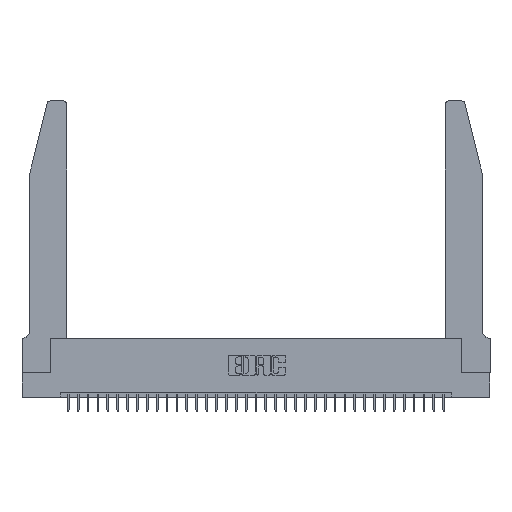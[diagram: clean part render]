
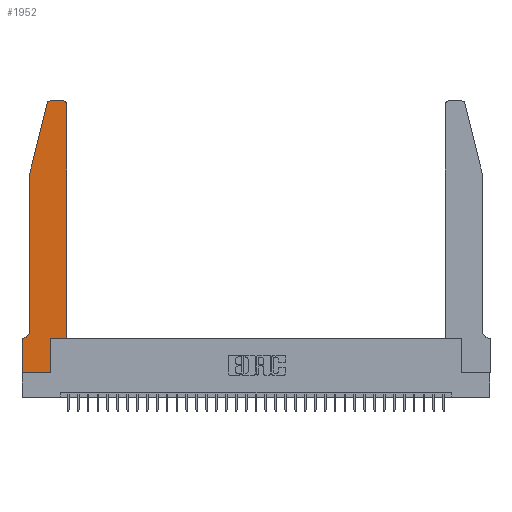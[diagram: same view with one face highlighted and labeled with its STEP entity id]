
A CAD part, top view. The second image highlights one B-rep face of the part: STEP entity #1952.
In plain terms, the highlighted planar face has unit normal (0, 0, 1).
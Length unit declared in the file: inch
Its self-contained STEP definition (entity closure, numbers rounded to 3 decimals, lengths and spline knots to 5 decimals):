
#158 = DIRECTION ( 'NONE',  ( 0., 0., -1. ) ) ;
#1492 = VECTOR ( 'NONE', #25824, 39.37008 ) ;
#1546 = CARTESIAN_POINT ( 'NONE',  ( 0.4505, 0.35, 0.37 ) ) ;
#1723 = LINE ( 'NONE', #1546, #2317 ) ;
#1856 = AXIS2_PLACEMENT_3D ( 'NONE', #34117, #3995, #17413 ) ;
#1952 = ADVANCED_FACE ( 'NONE', ( #29750 ), #30440, .T. ) ;
#2241 = DIRECTION ( 'NONE',  ( -1., 0., 0. ) ) ;
#2317 = VECTOR ( 'NONE', #34607, 39.37008 ) ;
#2616 = EDGE_CURVE ( 'NONE', #30620, #25859, #33422, .T. ) ;
#2762 = AXIS2_PLACEMENT_3D ( 'NONE', #13038, #24094, #8824 ) ;
#3745 = EDGE_CURVE ( 'NONE', #15324, #7167, #34876, .T. ) ;
#3892 = ORIENTED_EDGE ( 'NONE', *, *, #27287, .T. ) ;
#3995 = DIRECTION ( 'NONE',  ( 0., 0., 1. ) ) ;
#4018 = ORIENTED_EDGE ( 'NONE', *, *, #30330, .T. ) ;
#4283 = DIRECTION ( 'NONE',  ( 0., -1., 0. ) ) ;
#4850 = VERTEX_POINT ( 'NONE', #19926 ) ;
#4927 = CARTESIAN_POINT ( 'NONE',  ( 0.0055, 0.35, 0.37 ) ) ;
#5542 = DIRECTION ( 'NONE',  ( 0., 0., 1. ) ) ;
#5621 = DIRECTION ( 'NONE',  ( 0., 1., 0. ) ) ;
#5966 = DIRECTION ( 'NONE',  ( -1., 0., 0. ) ) ;
#6791 = CARTESIAN_POINT ( 'NONE',  ( 0.4505, 0.35, 0.37 ) ) ;
#7167 = VERTEX_POINT ( 'NONE', #4927 ) ;
#7569 = VECTOR ( 'NONE', #5621, 39.37008 ) ;
#8710 = CARTESIAN_POINT ( 'NONE',  ( 0.0755, 2., 0.37 ) ) ;
#8824 = DIRECTION ( 'NONE',  ( 1., 0., 0. ) ) ;
#9151 = CARTESIAN_POINT ( 'NONE',  ( 0., 0.35, 0.37 ) ) ;
#9332 = DIRECTION ( 'NONE',  ( 1., 0., 0. ) ) ;
#10185 = VECTOR ( 'NONE', #24872, 39.37008 ) ;
#10247 = ORIENTED_EDGE ( 'NONE', *, *, #20597, .T. ) ;
#10715 = EDGE_CURVE ( 'NONE', #7167, #22431, #14595, .T. ) ;
#11052 = VECTOR ( 'NONE', #28286, 39.37008 ) ;
#11178 = CARTESIAN_POINT ( 'NONE',  ( 0.25487, 2.72718, 0.37 ) ) ;
#11275 = CARTESIAN_POINT ( 'NONE',  ( 0.0755, 0.42, 0.37 ) ) ;
#13038 = CARTESIAN_POINT ( 'NONE',  ( 0.4205, 2.72, 0.37 ) ) ;
#14363 = CARTESIAN_POINT ( 'NONE',  ( 0.2865, 0.35, 0.37 ) ) ;
#14595 = LINE ( 'NONE', #31275, #1492 ) ;
#14712 = CARTESIAN_POINT ( 'NONE',  ( 0.284, 2.75, 0.37 ) ) ;
#14796 = CARTESIAN_POINT ( 'NONE',  ( 0., 0., 0.37 ) ) ;
#15324 = VERTEX_POINT ( 'NONE', #11275 ) ;
#15760 = VECTOR ( 'NONE', #2241, 39.37008 ) ;
#16419 = LINE ( 'NONE', #29851, #15760 ) ;
#16711 = EDGE_CURVE ( 'NONE', #26200, #34934, #25605, .T. ) ;
#16715 = ORIENTED_EDGE ( 'NONE', *, *, #2616, .T. ) ;
#16938 = CARTESIAN_POINT ( 'NONE',  ( 0.2865, 0., 0.37 ) ) ;
#17125 = EDGE_CURVE ( 'NONE', #22431, #19661, #30995, .T. ) ;
#17206 = CARTESIAN_POINT ( 'NONE',  ( 0., 0., 0.37 ) ) ;
#17397 = VERTEX_POINT ( 'NONE', #17517 ) ;
#17402 = CARTESIAN_POINT ( 'NONE',  ( 0.0055, 0.42, 0.37 ) ) ;
#17413 = DIRECTION ( 'NONE',  ( 1., 0., 0. ) ) ;
#17517 = CARTESIAN_POINT ( 'NONE',  ( 0.4205, 2.75, 0.37 ) ) ;
#18034 = DIRECTION ( 'NONE',  ( 0., 1., 0. ) ) ;
#19219 = EDGE_LOOP ( 'NONE', ( #24117, #26201, #3892, #24515, #34121, #21373, #25740, #23412, #16715, #27378, #10247, #4018 ) ) ;
#19345 = CARTESIAN_POINT ( 'NONE',  ( 0., 0.35, 0.37 ) ) ;
#19591 = LINE ( 'NONE', #8710, #10185 ) ;
#19661 = VERTEX_POINT ( 'NONE', #35707 ) ;
#19926 = CARTESIAN_POINT ( 'NONE',  ( 0.4505, 2.72, 0.37 ) ) ;
#20597 = EDGE_CURVE ( 'NONE', #30998, #4850, #24017, .T. ) ;
#20630 = LINE ( 'NONE', #20986, #28875 ) ;
#20851 = EDGE_CURVE ( 'NONE', #17397, #26200, #16419, .T. ) ;
#20986 = CARTESIAN_POINT ( 'NONE',  ( 0.0755, 2., 0.37 ) ) ;
#21373 = ORIENTED_EDGE ( 'NONE', *, *, #10715, .T. ) ;
#22431 = VERTEX_POINT ( 'NONE', #9151 ) ;
#22945 = LINE ( 'NONE', #14796, #34600 ) ;
#23412 = ORIENTED_EDGE ( 'NONE', *, *, #29116, .T. ) ;
#24017 = LINE ( 'NONE', #6791, #24435 ) ;
#24063 = CARTESIAN_POINT ( 'NONE',  ( 0.4505, 0.35, 0.37 ) ) ;
#24094 = DIRECTION ( 'NONE',  ( 0., 0., 1. ) ) ;
#24117 = ORIENTED_EDGE ( 'NONE', *, *, #20851, .T. ) ;
#24435 = VECTOR ( 'NONE', #18034, 39.37008 ) ;
#24515 = ORIENTED_EDGE ( 'NONE', *, *, #34141, .T. ) ;
#24793 = DIRECTION ( 'NONE',  ( 1., 0., 0. ) ) ;
#24872 = DIRECTION ( 'NONE',  ( -0.239, -0.971, 0. ) ) ;
#25605 = CIRCLE ( 'NONE', #1856, 0.03 ) ;
#25740 = ORIENTED_EDGE ( 'NONE', *, *, #17125, .T. ) ;
#25824 = DIRECTION ( 'NONE',  ( -1., 0., 0. ) ) ;
#25859 = VERTEX_POINT ( 'NONE', #29636 ) ;
#26200 = VERTEX_POINT ( 'NONE', #14712 ) ;
#26201 = ORIENTED_EDGE ( 'NONE', *, *, #16711, .T. ) ;
#27107 = CARTESIAN_POINT ( 'NONE',  ( 0.0755, 2., 0.37 ) ) ;
#27287 = EDGE_CURVE ( 'NONE', #34934, #33219, #19591, .T. ) ;
#27378 = ORIENTED_EDGE ( 'NONE', *, *, #31236, .T. ) ;
#28286 = DIRECTION ( 'NONE',  ( 0., -1., 0. ) ) ;
#28489 = AXIS2_PLACEMENT_3D ( 'NONE', #17402, #158, #5966 ) ;
#28875 = VECTOR ( 'NONE', #4283, 39.37008 ) ;
#29116 = EDGE_CURVE ( 'NONE', #19661, #30620, #22945, .T. ) ;
#29636 = CARTESIAN_POINT ( 'NONE',  ( 0.2865, 0.35, 0.37 ) ) ;
#29750 = FACE_OUTER_BOUND ( 'NONE', #19219, .T. ) ;
#29851 = CARTESIAN_POINT ( 'NONE',  ( 0.2605, 2.75, 0.37 ) ) ;
#30330 = EDGE_CURVE ( 'NONE', #4850, #17397, #34063, .T. ) ;
#30440 = PLANE ( 'NONE',  #35147 ) ;
#30620 = VERTEX_POINT ( 'NONE', #16938 ) ;
#30995 = LINE ( 'NONE', #17206, #11052 ) ;
#30998 = VERTEX_POINT ( 'NONE', #24063 ) ;
#31236 = EDGE_CURVE ( 'NONE', #25859, #30998, #1723, .T. ) ;
#31275 = CARTESIAN_POINT ( 'NONE',  ( 0.0755, 0.35, 0.37 ) ) ;
#33219 = VERTEX_POINT ( 'NONE', #27107 ) ;
#33422 = LINE ( 'NONE', #14363, #7569 ) ;
#34063 = CIRCLE ( 'NONE', #2762, 0.03 ) ;
#34117 = CARTESIAN_POINT ( 'NONE',  ( 0.284, 2.72, 0.37 ) ) ;
#34121 = ORIENTED_EDGE ( 'NONE', *, *, #3745, .T. ) ;
#34141 = EDGE_CURVE ( 'NONE', #33219, #15324, #20630, .T. ) ;
#34600 = VECTOR ( 'NONE', #9332, 39.37008 ) ;
#34607 = DIRECTION ( 'NONE',  ( 1., 0., 0. ) ) ;
#34876 = CIRCLE ( 'NONE', #28489, 0.07 ) ;
#34934 = VERTEX_POINT ( 'NONE', #11178 ) ;
#35147 = AXIS2_PLACEMENT_3D ( 'NONE', #19345, #5542, #24793 ) ;
#35707 = CARTESIAN_POINT ( 'NONE',  ( 0., 0., 0.37 ) ) ;
